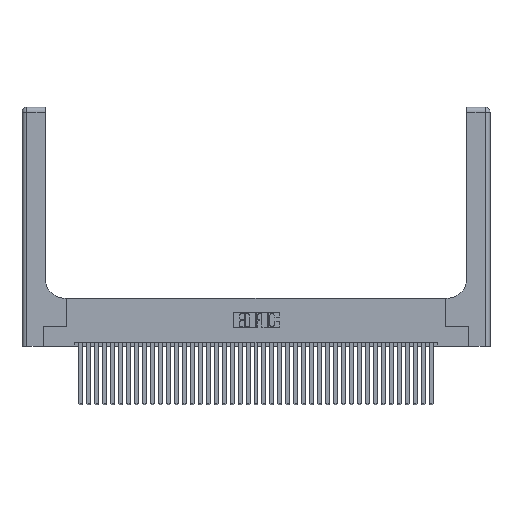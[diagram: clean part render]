
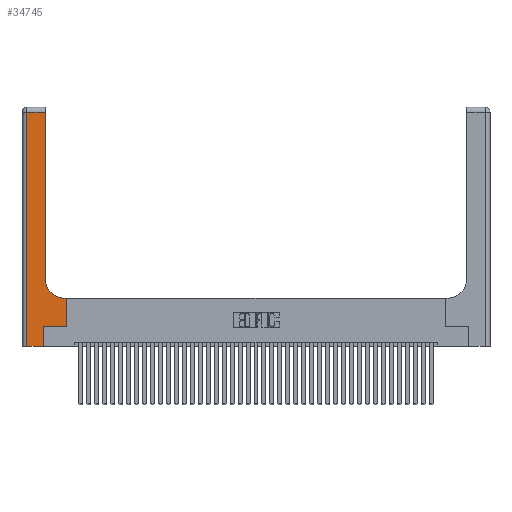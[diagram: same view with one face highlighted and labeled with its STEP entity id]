
A CAD part, top view. The second image highlights one B-rep face of the part: STEP entity #34745.
In plain terms, the highlighted planar face has unit normal (0, 0, 1).
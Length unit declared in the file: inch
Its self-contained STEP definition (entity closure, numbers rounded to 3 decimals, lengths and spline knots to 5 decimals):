
#1278 = ORIENTED_EDGE ( 'NONE', *, *, #1907, .T. ) ;
#1649 = DIRECTION ( 'NONE',  ( 0., 1., 0. ) ) ;
#1887 = DIRECTION ( 'NONE',  ( 0., 1., 0. ) ) ;
#1907 = EDGE_CURVE ( 'NONE', #36617, #7943, #2103, .T. ) ;
#2103 = LINE ( 'NONE', #4783, #9373 ) ;
#2566 = DIRECTION ( 'NONE',  ( 0., 0., -1. ) ) ;
#4314 = CARTESIAN_POINT ( 'NONE',  ( 0.269, 0.25, 0.37 ) ) ;
#4783 = CARTESIAN_POINT ( 'NONE',  ( 0.5585, 0.25, 0.37 ) ) ;
#5858 = LINE ( 'NONE', #30658, #37622 ) ;
#7422 = DIRECTION ( 'NONE',  ( 1., 0., 0. ) ) ;
#7626 = LINE ( 'NONE', #11831, #32203 ) ;
#7881 = EDGE_LOOP ( 'NONE', ( #20478, #16037, #25578, #28561, #27952, #21696, #1278, #20285, #31067 ) ) ;
#7943 = VERTEX_POINT ( 'NONE', #11608 ) ;
#8060 = DIRECTION ( 'NONE',  ( 0., -1., 0. ) ) ;
#9373 = VECTOR ( 'NONE', #1649, 39.37008 ) ;
#9713 = VECTOR ( 'NONE', #1887, 39.37008 ) ;
#10109 = DIRECTION ( 'NONE',  ( -1., 0., 0. ) ) ;
#10289 = CARTESIAN_POINT ( 'NONE',  ( 0.5415, 0.85, 0.37 ) ) ;
#10562 = VECTOR ( 'NONE', #15614, 39.37008 ) ;
#10607 = VECTOR ( 'NONE', #7422, 39.37008 ) ;
#11271 = VERTEX_POINT ( 'NONE', #17561 ) ;
#11608 = CARTESIAN_POINT ( 'NONE',  ( 0.5585, 0.6, 0.37 ) ) ;
#11831 = CARTESIAN_POINT ( 'NONE',  ( 0.269, 0., 0.37 ) ) ;
#12752 = EDGE_CURVE ( 'NONE', #7943, #30169, #35436, .T. ) ;
#12988 = VERTEX_POINT ( 'NONE', #20877 ) ;
#13389 = DIRECTION ( 'NONE',  ( 1., 0., 0. ) ) ;
#14113 = CARTESIAN_POINT ( 'NONE',  ( 0.06, 3., 0.37 ) ) ;
#14829 = VERTEX_POINT ( 'NONE', #21995 ) ;
#15134 = CARTESIAN_POINT ( 'NONE',  ( 0.5585, 0.25, 0.37 ) ) ;
#15614 = DIRECTION ( 'NONE',  ( -1., 0., 0. ) ) ;
#16037 = ORIENTED_EDGE ( 'NONE', *, *, #27223, .T. ) ;
#16178 = VECTOR ( 'NONE', #8060, 39.37008 ) ;
#16401 = CIRCLE ( 'NONE', #23829, 0.25 ) ;
#17040 = CARTESIAN_POINT ( 'NONE',  ( 0.5415, 0.6, 0.37 ) ) ;
#17152 = LINE ( 'NONE', #14113, #16178 ) ;
#17462 = AXIS2_PLACEMENT_3D ( 'NONE', #39479, #2566, #24196 ) ;
#17561 = CARTESIAN_POINT ( 'NONE',  ( 0.269, 0., 0.37 ) ) ;
#17906 = LINE ( 'NONE', #29556, #9713 ) ;
#17945 = PLANE ( 'NONE',  #17462 ) ;
#19896 = EDGE_CURVE ( 'NONE', #12988, #11271, #5858, .T. ) ;
#20122 = EDGE_CURVE ( 'NONE', #30169, #33071, #16401, .T. ) ;
#20285 = ORIENTED_EDGE ( 'NONE', *, *, #12752, .T. ) ;
#20478 = ORIENTED_EDGE ( 'NONE', *, *, #34628, .T. ) ;
#20877 = CARTESIAN_POINT ( 'NONE',  ( 0.06, 0., 0.37 ) ) ;
#21628 = CARTESIAN_POINT ( 'NONE',  ( 0.269, 0.25, 0.37 ) ) ;
#21696 = ORIENTED_EDGE ( 'NONE', *, *, #35546, .T. ) ;
#21995 = CARTESIAN_POINT ( 'NONE',  ( 0.2915, 2.94, 0.37 ) ) ;
#22098 = VERTEX_POINT ( 'NONE', #34774 ) ;
#22404 = CARTESIAN_POINT ( 'NONE',  ( 0.2915, 0.6, 0.37 ) ) ;
#22934 = EDGE_CURVE ( 'NONE', #22098, #12988, #17152, .T. ) ;
#23829 = AXIS2_PLACEMENT_3D ( 'NONE', #10289, #31840, #13389 ) ;
#24196 = DIRECTION ( 'NONE',  ( -1., 0., 0. ) ) ;
#24283 = DIRECTION ( 'NONE',  ( 0., 1., 0. ) ) ;
#25578 = ORIENTED_EDGE ( 'NONE', *, *, #22934, .T. ) ;
#25903 = VERTEX_POINT ( 'NONE', #21628 ) ;
#27025 = LINE ( 'NONE', #4314, #10607 ) ;
#27223 = EDGE_CURVE ( 'NONE', #14829, #22098, #35114, .T. ) ;
#27315 = VECTOR ( 'NONE', #10109, 39.37008 ) ;
#27717 = EDGE_CURVE ( 'NONE', #11271, #25903, #7626, .T. ) ;
#27926 = CARTESIAN_POINT ( 'NONE',  ( 0., 2.94, 0.37 ) ) ;
#27952 = ORIENTED_EDGE ( 'NONE', *, *, #27717, .T. ) ;
#28561 = ORIENTED_EDGE ( 'NONE', *, *, #19896, .T. ) ;
#29556 = CARTESIAN_POINT ( 'NONE',  ( 0.2915, 3., 0.37 ) ) ;
#30169 = VERTEX_POINT ( 'NONE', #17040 ) ;
#30658 = CARTESIAN_POINT ( 'NONE',  ( 0., 0., 0.37 ) ) ;
#31067 = ORIENTED_EDGE ( 'NONE', *, *, #20122, .T. ) ;
#31840 = DIRECTION ( 'NONE',  ( 0., 0., -1. ) ) ;
#32203 = VECTOR ( 'NONE', #24283, 39.37008 ) ;
#33071 = VERTEX_POINT ( 'NONE', #34218 ) ;
#34218 = CARTESIAN_POINT ( 'NONE',  ( 0.2915, 0.85, 0.37 ) ) ;
#34628 = EDGE_CURVE ( 'NONE', #33071, #14829, #17906, .T. ) ;
#34745 = ADVANCED_FACE ( 'NONE', ( #37643 ), #17945, .F. ) ;
#34774 = CARTESIAN_POINT ( 'NONE',  ( 0.06, 2.94, 0.37 ) ) ;
#35114 = LINE ( 'NONE', #27926, #10562 ) ;
#35436 = LINE ( 'NONE', #22404, #27315 ) ;
#35546 = EDGE_CURVE ( 'NONE', #25903, #36617, #27025, .T. ) ;
#36617 = VERTEX_POINT ( 'NONE', #15134 ) ;
#36949 = DIRECTION ( 'NONE',  ( 1., 0., 0. ) ) ;
#37622 = VECTOR ( 'NONE', #36949, 39.37008 ) ;
#37643 = FACE_OUTER_BOUND ( 'NONE', #7881, .T. ) ;
#39479 = CARTESIAN_POINT ( 'NONE',  ( 0., 3., 0.37 ) ) ;
